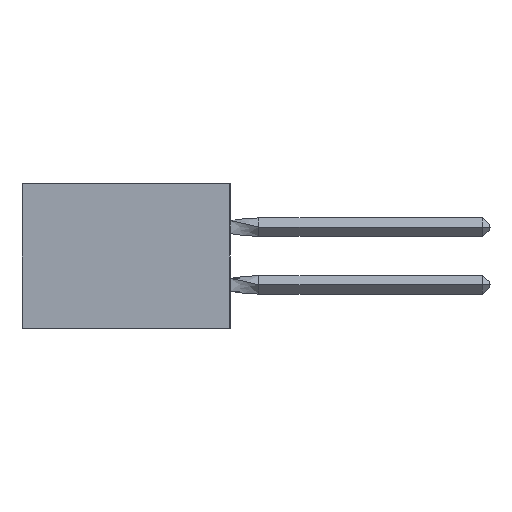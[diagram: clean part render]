
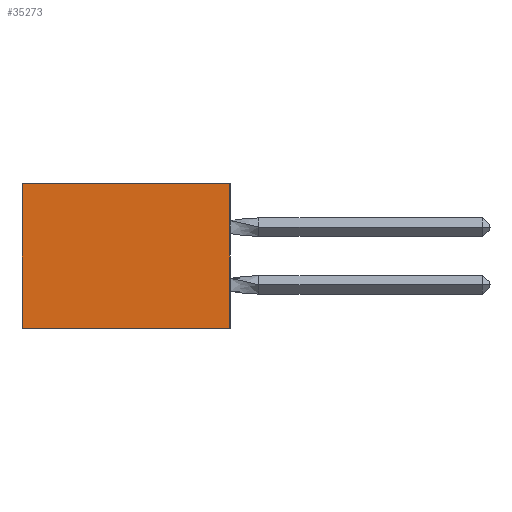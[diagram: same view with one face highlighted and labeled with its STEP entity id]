
A CAD part, left-side view. The second image highlights one B-rep face of the part: STEP entity #35273.
In plain terms, the highlighted planar face has unit normal (-1, 0, 0).
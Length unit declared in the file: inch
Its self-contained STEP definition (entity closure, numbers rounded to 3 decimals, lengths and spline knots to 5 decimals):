
#13 = CARTESIAN_POINT ( 'NONE',  ( 0.305, 0., -0.5 ) ) ;
#224 = VECTOR ( 'NONE', #9162, 39.37008 ) ;
#361 = DIRECTION ( 'NONE',  ( 0., 1., 0. ) ) ;
#952 = VECTOR ( 'NONE', #13973, 39.37008 ) ;
#1018 = EDGE_CURVE ( 'NONE', #27561, #23162, #30767, .T. ) ;
#1561 = CARTESIAN_POINT ( 'NONE',  ( 0.305, 0.72, 0. ) ) ;
#3880 = DIRECTION ( 'NONE',  ( 0., 0., -1. ) ) ;
#4614 = VERTEX_POINT ( 'NONE', #6762 ) ;
#6762 = CARTESIAN_POINT ( 'NONE',  ( 0.305, 0., -0.5 ) ) ;
#7037 = VECTOR ( 'NONE', #7937, 39.37008 ) ;
#7937 = DIRECTION ( 'NONE',  ( 0., 0., -1. ) ) ;
#8960 = AXIS2_PLACEMENT_3D ( 'NONE', #12939, #28594, #3880 ) ;
#9162 = DIRECTION ( 'NONE',  ( 0., 0., -1. ) ) ;
#12168 = EDGE_CURVE ( 'NONE', #4614, #23162, #14759, .T. ) ;
#12939 = CARTESIAN_POINT ( 'NONE',  ( 0.305, 0., -0.5 ) ) ;
#13520 = EDGE_CURVE ( 'NONE', #23673, #4614, #33028, .T. ) ;
#13973 = DIRECTION ( 'NONE',  ( 0., 1., 0. ) ) ;
#14759 = LINE ( 'NONE', #34716, #952 ) ;
#14790 = FACE_OUTER_BOUND ( 'NONE', #28905, .T. ) ;
#16268 = PLANE ( 'NONE',  #8960 ) ;
#18806 = ORIENTED_EDGE ( 'NONE', *, *, #25785, .T. ) ;
#20218 = CARTESIAN_POINT ( 'NONE',  ( 0.305, 0., 0. ) ) ;
#21372 = CARTESIAN_POINT ( 'NONE',  ( 0.305, 0., 0. ) ) ;
#23162 = VERTEX_POINT ( 'NONE', #27216 ) ;
#23673 = VERTEX_POINT ( 'NONE', #20218 ) ;
#25785 = EDGE_CURVE ( 'NONE', #23673, #27561, #30789, .T. ) ;
#26471 = VECTOR ( 'NONE', #361, 39.37008 ) ;
#27216 = CARTESIAN_POINT ( 'NONE',  ( 0.305, 0.72, -0.5 ) ) ;
#27544 = ORIENTED_EDGE ( 'NONE', *, *, #1018, .T. ) ;
#27561 = VERTEX_POINT ( 'NONE', #1561 ) ;
#28594 = DIRECTION ( 'NONE',  ( 1., 0., 0. ) ) ;
#28905 = EDGE_LOOP ( 'NONE', ( #27544, #35074, #31039, #18806 ) ) ;
#30767 = LINE ( 'NONE', #38353, #7037 ) ;
#30789 = LINE ( 'NONE', #21372, #26471 ) ;
#31039 = ORIENTED_EDGE ( 'NONE', *, *, #13520, .F. ) ;
#33028 = LINE ( 'NONE', #13, #224 ) ;
#34716 = CARTESIAN_POINT ( 'NONE',  ( 0.305, 0., -0.5 ) ) ;
#35074 = ORIENTED_EDGE ( 'NONE', *, *, #12168, .F. ) ;
#35273 = ADVANCED_FACE ( 'NONE', ( #14790 ), #16268, .F. ) ;
#38353 = CARTESIAN_POINT ( 'NONE',  ( 0.305, 0.72, -0.5 ) ) ;
